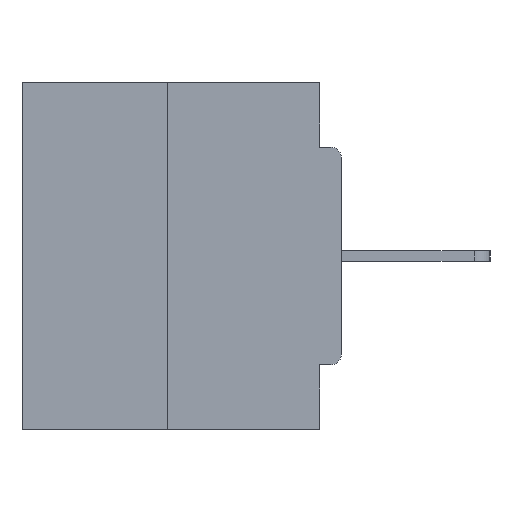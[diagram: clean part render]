
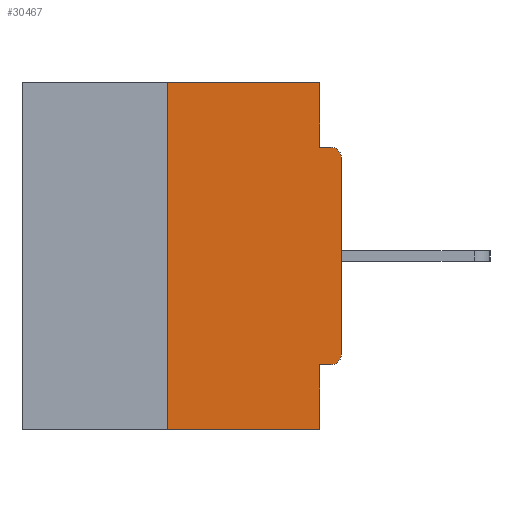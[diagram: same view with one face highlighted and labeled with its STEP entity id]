
A CAD part, left-side view. The second image highlights one B-rep face of the part: STEP entity #30467.
In plain terms, the highlighted planar face has unit normal (-1, 0, 0).
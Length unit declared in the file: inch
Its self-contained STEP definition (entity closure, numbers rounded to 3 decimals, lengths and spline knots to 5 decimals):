
#390 = VERTEX_POINT ( 'NONE', #21168 ) ;
#399 = LINE ( 'NONE', #14217, #18942 ) ;
#450 = EDGE_CURVE ( 'NONE', #12513, #19094, #901, .T. ) ;
#751 = ORIENTED_EDGE ( 'NONE', *, *, #22882, .T. ) ;
#901 = CIRCLE ( 'NONE', #5470, 0.015 ) ;
#1028 = CARTESIAN_POINT ( 'NONE',  ( 0., 0.031, 0. ) ) ;
#1852 = VERTEX_POINT ( 'NONE', #19796 ) ;
#1920 = ORIENTED_EDGE ( 'NONE', *, *, #19833, .F. ) ;
#2095 = EDGE_CURVE ( 'NONE', #10309, #1852, #399, .T. ) ;
#2637 = EDGE_LOOP ( 'NONE', ( #30364, #1920, #21028, #2710, #23157, #17821, #751, #7358, #17456, #6983 ) ) ;
#2710 = ORIENTED_EDGE ( 'NONE', *, *, #13607, .F. ) ;
#2810 = CARTESIAN_POINT ( 'NONE',  ( 0., 0.031, -0.5 ) ) ;
#2907 = VECTOR ( 'NONE', #17919, 39.37008 ) ;
#2978 = DIRECTION ( 'NONE',  ( 0., 0., -1. ) ) ;
#3552 = CARTESIAN_POINT ( 'NONE',  ( 0., 0.25, -0.5 ) ) ;
#3569 = DIRECTION ( 'NONE',  ( 0., 0., -1. ) ) ;
#4276 = VECTOR ( 'NONE', #6182, 39.37008 ) ;
#5049 = DIRECTION ( 'NONE',  ( -1., 0., 0. ) ) ;
#5089 = CARTESIAN_POINT ( 'NONE',  ( 0., 0.015, -0.3915 ) ) ;
#5170 = FACE_OUTER_BOUND ( 'NONE', #2637, .T. ) ;
#5470 = AXIS2_PLACEMENT_3D ( 'NONE', #5089, #5049, #2978 ) ;
#5845 = CARTESIAN_POINT ( 'NONE',  ( 0., 0.25, 0. ) ) ;
#6182 = DIRECTION ( 'NONE',  ( 0., -1., 0. ) ) ;
#6983 = ORIENTED_EDGE ( 'NONE', *, *, #8742, .F. ) ;
#7111 = EDGE_CURVE ( 'NONE', #12513, #10246, #26679, .T. ) ;
#7358 = ORIENTED_EDGE ( 'NONE', *, *, #10217, .T. ) ;
#7980 = VECTOR ( 'NONE', #13143, 39.37008 ) ;
#8742 = EDGE_CURVE ( 'NONE', #1852, #11359, #20088, .T. ) ;
#9694 = DIRECTION ( 'NONE',  ( -1., 0., 0. ) ) ;
#10217 = EDGE_CURVE ( 'NONE', #20411, #11916, #14163, .T. ) ;
#10246 = VERTEX_POINT ( 'NONE', #30510 ) ;
#10273 = CARTESIAN_POINT ( 'NONE',  ( 0., 0.015, -0.4065 ) ) ;
#10309 = VERTEX_POINT ( 'NONE', #21765 ) ;
#10786 = LINE ( 'NONE', #24977, #4276 ) ;
#11109 = DIRECTION ( 'NONE',  ( 0., 0., -1. ) ) ;
#11359 = VERTEX_POINT ( 'NONE', #24297 ) ;
#11380 = VECTOR ( 'NONE', #27201, 39.37008 ) ;
#11602 = AXIS2_PLACEMENT_3D ( 'NONE', #23665, #9694, #26043 ) ;
#11916 = VERTEX_POINT ( 'NONE', #14679 ) ;
#11996 = VECTOR ( 'NONE', #23986, 39.37008 ) ;
#12513 = VERTEX_POINT ( 'NONE', #10273 ) ;
#13135 = CARTESIAN_POINT ( 'NONE',  ( 0., 0., -0.4065 ) ) ;
#13143 = DIRECTION ( 'NONE',  ( 0., 1., 0. ) ) ;
#13194 = VECTOR ( 'NONE', #3569, 39.37008 ) ;
#13607 = EDGE_CURVE ( 'NONE', #10246, #390, #29501, .T. ) ;
#13612 = CARTESIAN_POINT ( 'NONE',  ( 0., 0., -0.1085 ) ) ;
#14163 = CIRCLE ( 'NONE', #11602, 0.015 ) ;
#14217 = CARTESIAN_POINT ( 'NONE',  ( 0., 0.46, 0. ) ) ;
#14679 = CARTESIAN_POINT ( 'NONE',  ( 0., 0.015, -0.0935 ) ) ;
#15791 = CARTESIAN_POINT ( 'NONE',  ( 0., 0.46, 0. ) ) ;
#16732 = EDGE_CURVE ( 'NONE', #25855, #390, #10786, .T. ) ;
#16894 = DIRECTION ( 'NONE',  ( 0., -1., 0. ) ) ;
#17456 = ORIENTED_EDGE ( 'NONE', *, *, #25071, .F. ) ;
#17658 = LINE ( 'NONE', #22349, #11380 ) ;
#17821 = ORIENTED_EDGE ( 'NONE', *, *, #450, .T. ) ;
#17919 = DIRECTION ( 'NONE',  ( 0., 0., 1. ) ) ;
#18942 = VECTOR ( 'NONE', #16894, 39.37008 ) ;
#19094 = VERTEX_POINT ( 'NONE', #26604 ) ;
#19796 = CARTESIAN_POINT ( 'NONE',  ( 0., 0.031, 0. ) ) ;
#19833 = EDGE_CURVE ( 'NONE', #25855, #10309, #28753, .T. ) ;
#20088 = LINE ( 'NONE', #1028, #13194 ) ;
#20411 = VERTEX_POINT ( 'NONE', #13612 ) ;
#21028 = ORIENTED_EDGE ( 'NONE', *, *, #16732, .T. ) ;
#21168 = CARTESIAN_POINT ( 'NONE',  ( 0., 0.031, -0.5 ) ) ;
#21580 = CARTESIAN_POINT ( 'NONE',  ( 0., 0., -0.0935 ) ) ;
#21765 = CARTESIAN_POINT ( 'NONE',  ( 0., 0.25, 0. ) ) ;
#21859 = DIRECTION ( 'NONE',  ( 0., 0., -1. ) ) ;
#22349 = CARTESIAN_POINT ( 'NONE',  ( 0., 0., 0. ) ) ;
#22706 = PLANE ( 'NONE',  #27951 ) ;
#22882 = EDGE_CURVE ( 'NONE', #19094, #20411, #17658, .T. ) ;
#23157 = ORIENTED_EDGE ( 'NONE', *, *, #7111, .F. ) ;
#23585 = LINE ( 'NONE', #21580, #11996 ) ;
#23665 = CARTESIAN_POINT ( 'NONE',  ( 0., 0.015, -0.1085 ) ) ;
#23986 = DIRECTION ( 'NONE',  ( 0., -1., 0. ) ) ;
#24297 = CARTESIAN_POINT ( 'NONE',  ( 0., 0.031, -0.0935 ) ) ;
#24977 = CARTESIAN_POINT ( 'NONE',  ( 0., 0.46, -0.5 ) ) ;
#25071 = EDGE_CURVE ( 'NONE', #11359, #11916, #23585, .T. ) ;
#25081 = DIRECTION ( 'NONE',  ( 1., 0., 0. ) ) ;
#25855 = VERTEX_POINT ( 'NONE', #3552 ) ;
#26043 = DIRECTION ( 'NONE',  ( 0., 0., -1. ) ) ;
#26604 = CARTESIAN_POINT ( 'NONE',  ( 0., 0., -0.3915 ) ) ;
#26679 = LINE ( 'NONE', #13135, #7980 ) ;
#27201 = DIRECTION ( 'NONE',  ( 0., 0., 1. ) ) ;
#27951 = AXIS2_PLACEMENT_3D ( 'NONE', #15791, #25081, #11109 ) ;
#28753 = LINE ( 'NONE', #5845, #2907 ) ;
#28770 = VECTOR ( 'NONE', #21859, 39.37008 ) ;
#29501 = LINE ( 'NONE', #2810, #28770 ) ;
#30364 = ORIENTED_EDGE ( 'NONE', *, *, #2095, .F. ) ;
#30467 = ADVANCED_FACE ( 'NONE', ( #5170 ), #22706, .F. ) ;
#30510 = CARTESIAN_POINT ( 'NONE',  ( 0., 0.031, -0.4065 ) ) ;
